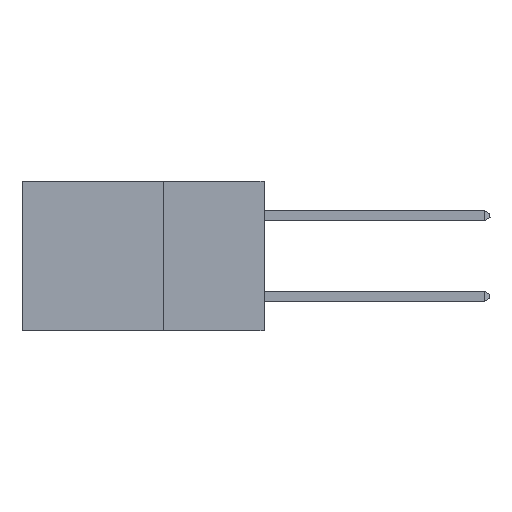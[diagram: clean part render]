
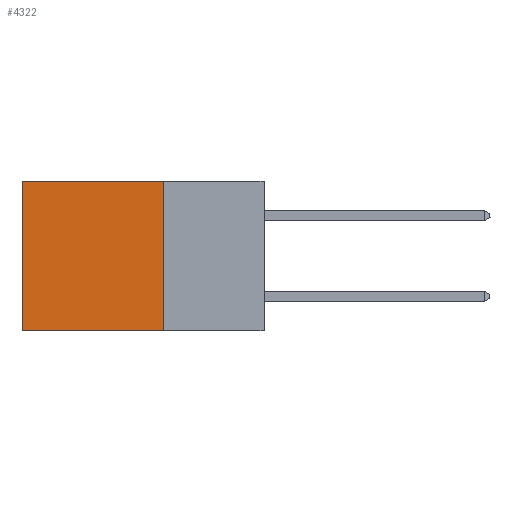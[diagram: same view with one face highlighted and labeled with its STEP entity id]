
A CAD part, left-side view. The second image highlights one B-rep face of the part: STEP entity #4322.
In plain terms, the highlighted planar face has unit normal (-1, 0, 0).
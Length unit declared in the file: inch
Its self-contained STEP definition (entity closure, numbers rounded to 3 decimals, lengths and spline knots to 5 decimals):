
#238 = EDGE_CURVE ( 'NONE', #926, #8718, #4665, .T. ) ;
#270 = VECTOR ( 'NONE', #13046, 39.37008 ) ;
#346 = VERTEX_POINT ( 'NONE', #14710 ) ;
#709 = LINE ( 'NONE', #10254, #270 ) ;
#913 = VECTOR ( 'NONE', #3376, 39.37008 ) ;
#926 = VERTEX_POINT ( 'NONE', #17014 ) ;
#1000 = EDGE_CURVE ( 'NONE', #13775, #926, #6819, .T. ) ;
#1078 = EDGE_LOOP ( 'NONE', ( #5546, #9254, #14741, #2578 ) ) ;
#1705 = AXIS2_PLACEMENT_3D ( 'NONE', #3584, #3519, #13372 ) ;
#1935 = CARTESIAN_POINT ( 'NONE',  ( 0.298, 0.25, 0. ) ) ;
#2578 = ORIENTED_EDGE ( 'NONE', *, *, #16208, .T. ) ;
#3376 = DIRECTION ( 'NONE',  ( 0., 1., 0. ) ) ;
#3519 = DIRECTION ( 'NONE',  ( 1., 0., 0. ) ) ;
#3584 = CARTESIAN_POINT ( 'NONE',  ( 0.298, 0.25, 0. ) ) ;
#3749 = DIRECTION ( 'NONE',  ( 0., 1., 0. ) ) ;
#4322 = ADVANCED_FACE ( 'NONE', ( #13206 ), #7602, .F. ) ;
#4665 = LINE ( 'NONE', #7396, #913 ) ;
#5546 = ORIENTED_EDGE ( 'NONE', *, *, #13709, .T. ) ;
#6340 = VECTOR ( 'NONE', #3749, 39.37008 ) ;
#6819 = LINE ( 'NONE', #6883, #12643 ) ;
#6883 = CARTESIAN_POINT ( 'NONE',  ( 0.298, 0.25, 0. ) ) ;
#7396 = CARTESIAN_POINT ( 'NONE',  ( 0.298, 0.25, -0.37 ) ) ;
#7602 = PLANE ( 'NONE',  #1705 ) ;
#8718 = VERTEX_POINT ( 'NONE', #13861 ) ;
#9254 = ORIENTED_EDGE ( 'NONE', *, *, #238, .F. ) ;
#10254 = CARTESIAN_POINT ( 'NONE',  ( 0.298, 0.6, 0. ) ) ;
#11415 = DIRECTION ( 'NONE',  ( 0., 0., -1. ) ) ;
#11733 = CARTESIAN_POINT ( 'NONE',  ( 0.298, 0.25, 0. ) ) ;
#12643 = VECTOR ( 'NONE', #11415, 39.37008 ) ;
#13046 = DIRECTION ( 'NONE',  ( 0., 0., -1. ) ) ;
#13206 = FACE_OUTER_BOUND ( 'NONE', #1078, .T. ) ;
#13372 = DIRECTION ( 'NONE',  ( 0., 0., -1. ) ) ;
#13709 = EDGE_CURVE ( 'NONE', #346, #8718, #709, .T. ) ;
#13775 = VERTEX_POINT ( 'NONE', #11733 ) ;
#13861 = CARTESIAN_POINT ( 'NONE',  ( 0.298, 0.6, -0.37 ) ) ;
#14129 = LINE ( 'NONE', #1935, #6340 ) ;
#14710 = CARTESIAN_POINT ( 'NONE',  ( 0.298, 0.6, 0. ) ) ;
#14741 = ORIENTED_EDGE ( 'NONE', *, *, #1000, .F. ) ;
#16208 = EDGE_CURVE ( 'NONE', #13775, #346, #14129, .T. ) ;
#17014 = CARTESIAN_POINT ( 'NONE',  ( 0.298, 0.25, -0.37 ) ) ;
